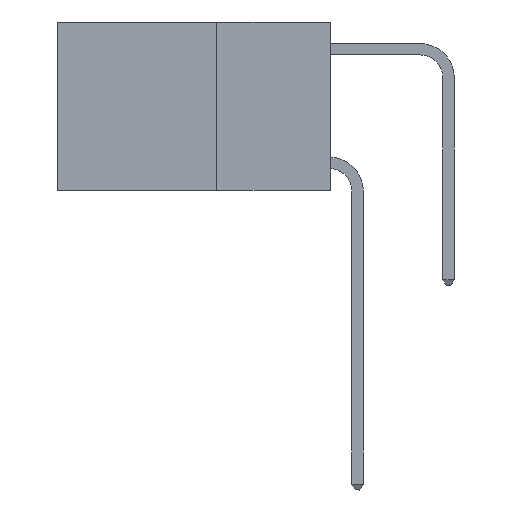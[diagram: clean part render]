
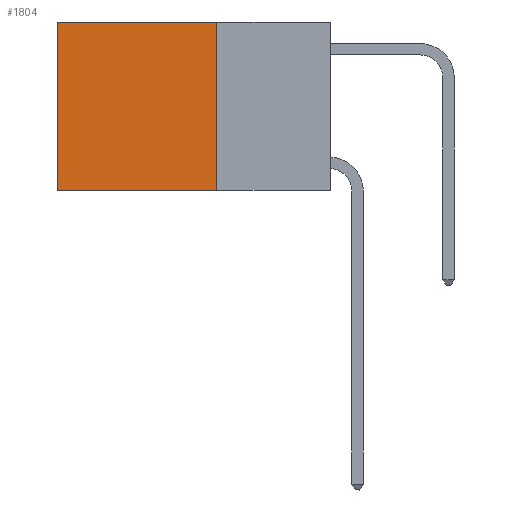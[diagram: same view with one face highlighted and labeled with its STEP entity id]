
A CAD part, left-side view. The second image highlights one B-rep face of the part: STEP entity #1804.
In plain terms, the highlighted planar face has unit normal (-1, 0, 0).
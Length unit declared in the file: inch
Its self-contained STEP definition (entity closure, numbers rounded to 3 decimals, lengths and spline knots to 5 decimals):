
#67 = EDGE_LOOP ( 'NONE', ( #8042, #11403, #7479, #10688 ) ) ;
#620 = LINE ( 'NONE', #5352, #7414 ) ;
#686 = CARTESIAN_POINT ( 'NONE',  ( 0.2625, 0.25, 0. ) ) ;
#860 = LINE ( 'NONE', #10289, #10361 ) ;
#1164 = EDGE_CURVE ( 'NONE', #6872, #5121, #620, .T. ) ;
#1466 = LINE ( 'NONE', #3694, #3993 ) ;
#1804 = ADVANCED_FACE ( 'NONE', ( #10546 ), #2762, .F. ) ;
#2061 = DIRECTION ( 'NONE',  ( 0., 0., -1. ) ) ;
#2276 = CARTESIAN_POINT ( 'NONE',  ( 0.2625, 0.6, -0.37 ) ) ;
#2361 = CARTESIAN_POINT ( 'NONE',  ( 0.2625, 0.25, -0.37 ) ) ;
#2594 = EDGE_CURVE ( 'NONE', #8516, #6872, #1466, .T. ) ;
#2762 = PLANE ( 'NONE',  #12184 ) ;
#2913 = DIRECTION ( 'NONE',  ( 0., 1., 0. ) ) ;
#2920 = VERTEX_POINT ( 'NONE', #2361 ) ;
#2927 = CARTESIAN_POINT ( 'NONE',  ( 0.2625, 0.25, 0. ) ) ;
#3694 = CARTESIAN_POINT ( 'NONE',  ( 0.2625, 0.25, 0. ) ) ;
#3993 = VECTOR ( 'NONE', #8539, 39.37008 ) ;
#4032 = DIRECTION ( 'NONE',  ( 1., 0., 0. ) ) ;
#4913 = CARTESIAN_POINT ( 'NONE',  ( 0.2625, 0.25, 0. ) ) ;
#5121 = VERTEX_POINT ( 'NONE', #2276 ) ;
#5352 = CARTESIAN_POINT ( 'NONE',  ( 0.2625, 0.6, 0. ) ) ;
#6425 = DIRECTION ( 'NONE',  ( 0., 0., -1. ) ) ;
#6872 = VERTEX_POINT ( 'NONE', #8804 ) ;
#7073 = LINE ( 'NONE', #686, #7088 ) ;
#7088 = VECTOR ( 'NONE', #6425, 39.37008 ) ;
#7414 = VECTOR ( 'NONE', #11154, 39.37008 ) ;
#7479 = ORIENTED_EDGE ( 'NONE', *, *, #11163, .F. ) ;
#8042 = ORIENTED_EDGE ( 'NONE', *, *, #1164, .T. ) ;
#8516 = VERTEX_POINT ( 'NONE', #4913 ) ;
#8539 = DIRECTION ( 'NONE',  ( 0., 1., 0. ) ) ;
#8804 = CARTESIAN_POINT ( 'NONE',  ( 0.2625, 0.6, 0. ) ) ;
#10289 = CARTESIAN_POINT ( 'NONE',  ( 0.2625, 0.25, -0.37 ) ) ;
#10361 = VECTOR ( 'NONE', #2913, 39.37008 ) ;
#10546 = FACE_OUTER_BOUND ( 'NONE', #67, .T. ) ;
#10688 = ORIENTED_EDGE ( 'NONE', *, *, #2594, .T. ) ;
#11154 = DIRECTION ( 'NONE',  ( 0., 0., -1. ) ) ;
#11163 = EDGE_CURVE ( 'NONE', #8516, #2920, #7073, .T. ) ;
#11289 = EDGE_CURVE ( 'NONE', #2920, #5121, #860, .T. ) ;
#11403 = ORIENTED_EDGE ( 'NONE', *, *, #11289, .F. ) ;
#12184 = AXIS2_PLACEMENT_3D ( 'NONE', #2927, #4032, #2061 ) ;
